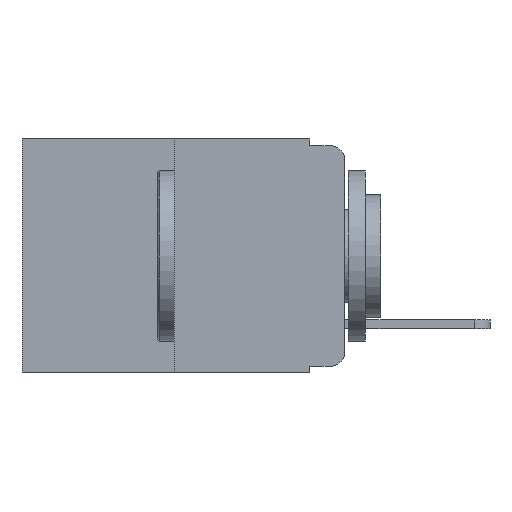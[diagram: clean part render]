
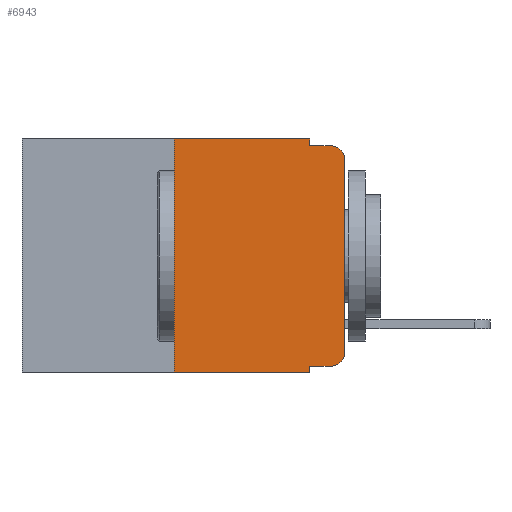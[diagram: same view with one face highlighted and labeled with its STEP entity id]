
A CAD part, left-side view. The second image highlights one B-rep face of the part: STEP entity #6943.
In plain terms, the highlighted planar face has unit normal (-1, 0, 0).
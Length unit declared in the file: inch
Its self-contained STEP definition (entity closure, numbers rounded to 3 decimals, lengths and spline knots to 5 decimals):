
#21 = LINE ( 'NONE', #951, #2284 ) ;
#71 = CARTESIAN_POINT ( 'NONE',  ( 0., 0.051, -0.343 ) ) ;
#108 = CIRCLE ( 'NONE', #2371, 0.02 ) ;
#429 = CARTESIAN_POINT ( 'NONE',  ( 0., 0.051, -0.333 ) ) ;
#551 = CARTESIAN_POINT ( 'NONE',  ( 0., 0.473, -0.343 ) ) ;
#593 = DIRECTION ( 'NONE',  ( 0., -1., 0. ) ) ;
#656 = EDGE_CURVE ( 'NONE', #820, #1181, #5794, .T. ) ;
#820 = VERTEX_POINT ( 'NONE', #3132 ) ;
#841 = DIRECTION ( 'NONE',  ( 0., 0., 1. ) ) ;
#901 = CARTESIAN_POINT ( 'NONE',  ( 0., 0.473, 0. ) ) ;
#917 = DIRECTION ( 'NONE',  ( 1., 0., 0. ) ) ;
#951 = CARTESIAN_POINT ( 'NONE',  ( 0., 0., 0. ) ) ;
#1181 = VERTEX_POINT ( 'NONE', #1478 ) ;
#1270 = DIRECTION ( 'NONE',  ( 0., 0., 1. ) ) ;
#1274 = VERTEX_POINT ( 'NONE', #7369 ) ;
#1441 = VERTEX_POINT ( 'NONE', #4654 ) ;
#1478 = CARTESIAN_POINT ( 'NONE',  ( 0., 0., -0.313 ) ) ;
#1556 = EDGE_CURVE ( 'NONE', #2053, #1441, #3144, .T. ) ;
#1787 = CARTESIAN_POINT ( 'NONE',  ( 0., 0.25, 0. ) ) ;
#1885 = DIRECTION ( 'NONE',  ( 0., -1., 0. ) ) ;
#1903 = ORIENTED_EDGE ( 'NONE', *, *, #2980, .T. ) ;
#2051 = ORIENTED_EDGE ( 'NONE', *, *, #6592, .T. ) ;
#2053 = VERTEX_POINT ( 'NONE', #3948 ) ;
#2167 = EDGE_CURVE ( 'NONE', #10089, #11082, #10533, .T. ) ;
#2168 = PLANE ( 'NONE',  #9105 ) ;
#2210 = ORIENTED_EDGE ( 'NONE', *, *, #9842, .F. ) ;
#2284 = VECTOR ( 'NONE', #1270, 39.37008 ) ;
#2371 = AXIS2_PLACEMENT_3D ( 'NONE', #2758, #2676, #9807 ) ;
#2475 = EDGE_CURVE ( 'NONE', #11082, #2053, #3124, .T. ) ;
#2482 = ORIENTED_EDGE ( 'NONE', *, *, #1556, .F. ) ;
#2563 = LINE ( 'NONE', #5159, #7015 ) ;
#2676 = DIRECTION ( 'NONE',  ( -1., 0., 0. ) ) ;
#2758 = CARTESIAN_POINT ( 'NONE',  ( 0., 0.02, -0.03 ) ) ;
#2910 = ORIENTED_EDGE ( 'NONE', *, *, #2475, .F. ) ;
#2980 = EDGE_CURVE ( 'NONE', #1181, #4642, #21, .T. ) ;
#3124 = LINE ( 'NONE', #5778, #7781 ) ;
#3132 = CARTESIAN_POINT ( 'NONE',  ( 0., 0.02, -0.333 ) ) ;
#3144 = LINE ( 'NONE', #4728, #9695 ) ;
#3175 = ORIENTED_EDGE ( 'NONE', *, *, #2167, .F. ) ;
#3184 = ORIENTED_EDGE ( 'NONE', *, *, #9826, .T. ) ;
#3304 = ORIENTED_EDGE ( 'NONE', *, *, #5787, .F. ) ;
#3439 = ORIENTED_EDGE ( 'NONE', *, *, #11197, .T. ) ;
#3712 = ORIENTED_EDGE ( 'NONE', *, *, #656, .T. ) ;
#3908 = DIRECTION ( 'NONE',  ( 0., 0., -1. ) ) ;
#3948 = CARTESIAN_POINT ( 'NONE',  ( 0., 0.051, 0. ) ) ;
#4324 = DIRECTION ( 'NONE',  ( -1., 0., 0. ) ) ;
#4388 = DIRECTION ( 'NONE',  ( 0., 0., -1. ) ) ;
#4600 = CARTESIAN_POINT ( 'NONE',  ( 0., 0.25, -0.343 ) ) ;
#4642 = VERTEX_POINT ( 'NONE', #8337 ) ;
#4654 = CARTESIAN_POINT ( 'NONE',  ( 0., 0.051, -0.01 ) ) ;
#4655 = VECTOR ( 'NONE', #1885, 39.37008 ) ;
#4728 = CARTESIAN_POINT ( 'NONE',  ( 0., 0.051, 0. ) ) ;
#4955 = VECTOR ( 'NONE', #5117, 39.37008 ) ;
#5117 = DIRECTION ( 'NONE',  ( 0., -1., 0. ) ) ;
#5134 = VERTEX_POINT ( 'NONE', #71 ) ;
#5159 = CARTESIAN_POINT ( 'NONE',  ( 0., 0.051, -0.01 ) ) ;
#5700 = DIRECTION ( 'NONE',  ( 0., -1., 0. ) ) ;
#5757 = DIRECTION ( 'NONE',  ( 0., 0., -1. ) ) ;
#5778 = CARTESIAN_POINT ( 'NONE',  ( 0., 0.473, 0. ) ) ;
#5787 = EDGE_CURVE ( 'NONE', #5852, #5134, #8227, .T. ) ;
#5794 = CIRCLE ( 'NONE', #10574, 0.02 ) ;
#5852 = VERTEX_POINT ( 'NONE', #429 ) ;
#5857 = FACE_OUTER_BOUND ( 'NONE', #6843, .T. ) ;
#6036 = CARTESIAN_POINT ( 'NONE',  ( 0., 0.02, -0.313 ) ) ;
#6234 = VECTOR ( 'NONE', #841, 39.37008 ) ;
#6592 = EDGE_CURVE ( 'NONE', #4642, #1274, #108, .T. ) ;
#6843 = EDGE_LOOP ( 'NONE', ( #1903, #2051, #2210, #2482, #2910, #3175, #3184, #3304, #3439, #3712 ) ) ;
#6943 = ADVANCED_FACE ( 'NONE', ( #5857 ), #2168, .F. ) ;
#6982 = CARTESIAN_POINT ( 'NONE',  ( 0., 0.25, 0. ) ) ;
#7015 = VECTOR ( 'NONE', #593, 39.37008 ) ;
#7255 = LINE ( 'NONE', #10372, #4655 ) ;
#7369 = CARTESIAN_POINT ( 'NONE',  ( 0., 0.02, -0.01 ) ) ;
#7532 = LINE ( 'NONE', #551, #4955 ) ;
#7781 = VECTOR ( 'NONE', #5700, 39.37008 ) ;
#8227 = LINE ( 'NONE', #8697, #9860 ) ;
#8337 = CARTESIAN_POINT ( 'NONE',  ( 0., 0., -0.03 ) ) ;
#8356 = DIRECTION ( 'NONE',  ( 0., 0., -1. ) ) ;
#8697 = CARTESIAN_POINT ( 'NONE',  ( 0., 0.051, 0. ) ) ;
#9105 = AXIS2_PLACEMENT_3D ( 'NONE', #901, #917, #5757 ) ;
#9695 = VECTOR ( 'NONE', #3908, 39.37008 ) ;
#9807 = DIRECTION ( 'NONE',  ( 0., 0., -1. ) ) ;
#9826 = EDGE_CURVE ( 'NONE', #10089, #5134, #7532, .T. ) ;
#9842 = EDGE_CURVE ( 'NONE', #1441, #1274, #2563, .T. ) ;
#9860 = VECTOR ( 'NONE', #8356, 39.37008 ) ;
#10089 = VERTEX_POINT ( 'NONE', #4600 ) ;
#10372 = CARTESIAN_POINT ( 'NONE',  ( 0., 0.051, -0.333 ) ) ;
#10533 = LINE ( 'NONE', #1787, #6234 ) ;
#10574 = AXIS2_PLACEMENT_3D ( 'NONE', #6036, #4324, #4388 ) ;
#11082 = VERTEX_POINT ( 'NONE', #6982 ) ;
#11197 = EDGE_CURVE ( 'NONE', #5852, #820, #7255, .T. ) ;
